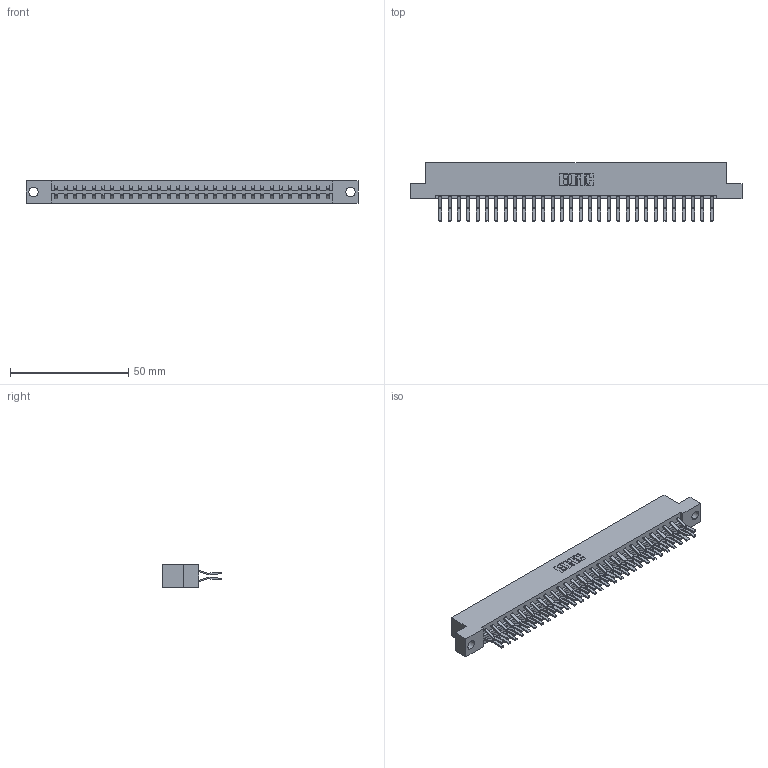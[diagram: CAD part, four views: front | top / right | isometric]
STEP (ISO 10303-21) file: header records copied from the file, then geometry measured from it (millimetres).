
FILE_DESCRIPTION (( 'STEP AP203' ), '1' );
FILE_NAME ('333-060-560-204.STEP', '2018-08-04T07:54:00', ( '' ), ( '' ), 'SwSTEP 2.0', 'SolidWorks 2016', '' );
FILE_SCHEMA (( 'CONFIG_CONTROL_DESIGN' ));
Length unit declared in the file: inch
Products named in the file (3): 333 Part_Flush - .156 Dia - TH; 345-292-001_560 Tail; 333-060-560-204
Assembly tree (61 placements, depth 2):
  333-060-560-204
    333 Part_Flush - .156 Dia - TH
    345-292-001_560 Tail  x60
Bounding box: 140.41 x 24.78 x 9.4 mm (x, y, z)
Volume: 14528.4 mm3; surface area: 17968.5 mm2
Topology: 61 solids, 61 shells, 3354 faces, 9971 edges, 6566 vertices
Faces by surface type: plane 2230, cylinder 1124
Entity records: 20943 total; most frequent: CARTESIAN_POINT 3486, ORIENTED_EDGE 3422, DIRECTION 3003, EDGE_CURVE 1711, LINE 1579, VECTOR 1579, VERTEX_POINT 1138, AXIS2_PLACEMENT_3D 712
